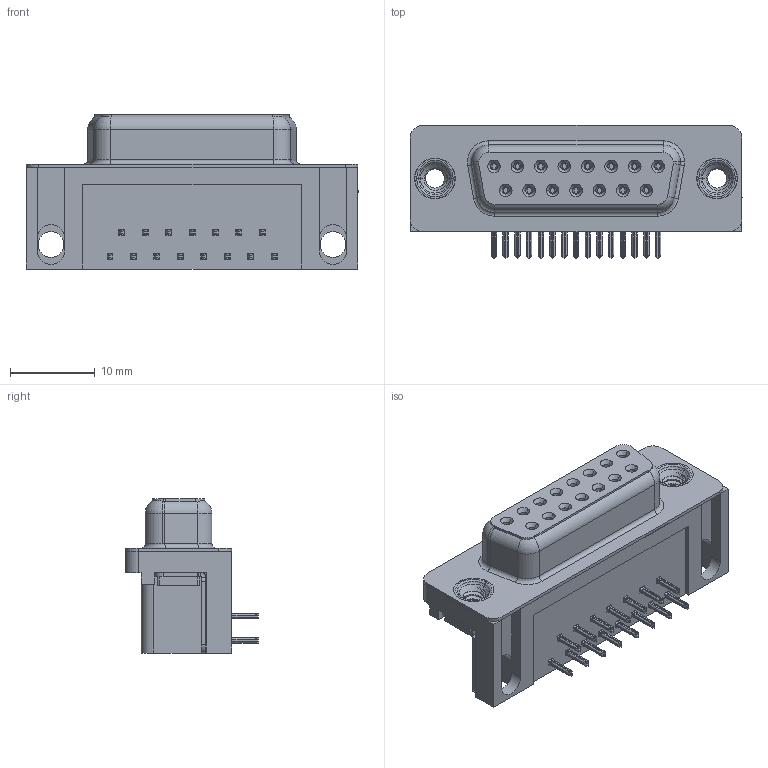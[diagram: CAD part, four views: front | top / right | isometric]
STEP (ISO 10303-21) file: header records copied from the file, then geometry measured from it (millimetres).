
FILE_DESCRIPTION (( 'STEP AP203' ), '1' );
FILE_NAME ('622-015-268-512.STEP', '2019-11-19T23:02:09', ( '' ), ( '' ), 'SwSTEP 2.0', 'SolidWorks 2016', '' );
FILE_SCHEMA (( 'CONFIG_CONTROL_DESIGN' ));
Length unit declared in the file: millimetre
Products named in the file (7): 622 Thru Hole Board Mount; 622-015-268-512; 622 Shell_15 Socket; 622 Housing_15 Socket; 622 Contact Top; 622 Socket Bottom; 622 4-40 Threaded Rivet
Assembly tree (21 placements, depth 2):
  622-015-268-512
    622 Housing_15 Socket
    622 Shell_15 Socket
    622 Socket Bottom  x7
    622 Contact Top  x8
    622 Thru Hole Board Mount  x2
    622 4-40 Threaded Rivet  x2
Bounding box: 39.22 x 15.73 x 18.2 mm (x, y, z)
Volume: 5187.1 mm3; surface area: 6702.8 mm2
Topology: 21 solids, 21 shells, 2425 faces, 6364 edges, 3996 vertices
Faces by surface type: plane 1072, cylinder 605, bspline 518, cone 192, torus 38
Entity records: 26501 total; most frequent: CARTESIAN_POINT 9015, ORIENTED_EDGE 3532, DIRECTION 3154, EDGE_CURVE 1766, VERTEX_POINT 1124, VECTOR 1086, LINE 1086, AXIS2_PLACEMENT_3D 1034
